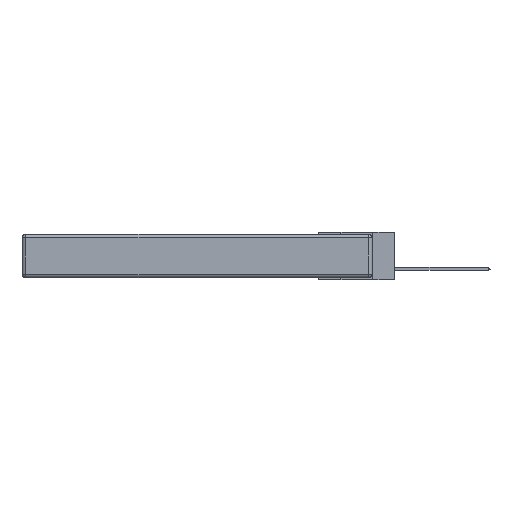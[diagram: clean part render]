
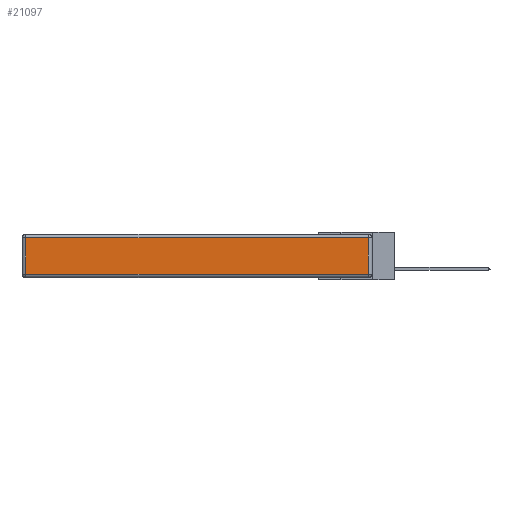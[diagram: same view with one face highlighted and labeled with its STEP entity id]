
A CAD part, left-side view. The second image highlights one B-rep face of the part: STEP entity #21097.
In plain terms, the highlighted planar face has unit normal (-1, 0, 0).
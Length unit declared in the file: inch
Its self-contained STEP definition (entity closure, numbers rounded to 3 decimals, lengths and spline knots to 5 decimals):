
#243 = EDGE_CURVE ( 'NONE', #16409, #22165, #5849, .T. ) ;
#747 = VERTEX_POINT ( 'NONE', #2492 ) ;
#1252 = AXIS2_PLACEMENT_3D ( 'NONE', #21568, #6762, #8653 ) ;
#2492 = CARTESIAN_POINT ( 'NONE',  ( 0., 0.03, -0.313 ) ) ;
#2910 = VECTOR ( 'NONE', #4854, 39.37008 ) ;
#4437 = CARTESIAN_POINT ( 'NONE',  ( 0., 0., -0.313 ) ) ;
#4854 = DIRECTION ( 'NONE',  ( 0., -1., 0. ) ) ;
#5485 = FACE_OUTER_BOUND ( 'NONE', #18201, .T. ) ;
#5849 = LINE ( 'NONE', #16202, #8765 ) ;
#6510 = CARTESIAN_POINT ( 'NONE',  ( 0., 2.75, -0.03 ) ) ;
#6762 = DIRECTION ( 'NONE',  ( -1., 0., 0. ) ) ;
#7307 = VECTOR ( 'NONE', #8206, 39.37008 ) ;
#8121 = ORIENTED_EDGE ( 'NONE', *, *, #243, .T. ) ;
#8206 = DIRECTION ( 'NONE',  ( 0., 0., 1. ) ) ;
#8380 = CARTESIAN_POINT ( 'NONE',  ( 0., 2.72, -0.313 ) ) ;
#8384 = EDGE_CURVE ( 'NONE', #22165, #747, #23804, .T. ) ;
#8400 = DIRECTION ( 'NONE',  ( 0., 1., 0. ) ) ;
#8653 = DIRECTION ( 'NONE',  ( 0., 0., 1. ) ) ;
#8765 = VECTOR ( 'NONE', #20094, 39.37008 ) ;
#10004 = EDGE_CURVE ( 'NONE', #747, #18647, #22603, .T. ) ;
#11236 = VECTOR ( 'NONE', #8400, 39.37008 ) ;
#13705 = CARTESIAN_POINT ( 'NONE',  ( 0., 0.03, -0.343 ) ) ;
#14139 = PLANE ( 'NONE',  #1252 ) ;
#15272 = ORIENTED_EDGE ( 'NONE', *, *, #8384, .T. ) ;
#16202 = CARTESIAN_POINT ( 'NONE',  ( 0., 2.72, -0.343 ) ) ;
#16280 = CARTESIAN_POINT ( 'NONE',  ( 0., 0.03, -0.03 ) ) ;
#16409 = VERTEX_POINT ( 'NONE', #20527 ) ;
#17378 = LINE ( 'NONE', #6510, #11236 ) ;
#17564 = EDGE_CURVE ( 'NONE', #18647, #16409, #17378, .T. ) ;
#17737 = ORIENTED_EDGE ( 'NONE', *, *, #17564, .T. ) ;
#18201 = EDGE_LOOP ( 'NONE', ( #15272, #19246, #17737, #8121 ) ) ;
#18647 = VERTEX_POINT ( 'NONE', #16280 ) ;
#19246 = ORIENTED_EDGE ( 'NONE', *, *, #10004, .T. ) ;
#20094 = DIRECTION ( 'NONE',  ( 0., 0., -1. ) ) ;
#20527 = CARTESIAN_POINT ( 'NONE',  ( 0., 2.72, -0.03 ) ) ;
#21097 = ADVANCED_FACE ( 'NONE', ( #5485 ), #14139, .T. ) ;
#21568 = CARTESIAN_POINT ( 'NONE',  ( 0., 0., -0.343 ) ) ;
#22165 = VERTEX_POINT ( 'NONE', #8380 ) ;
#22603 = LINE ( 'NONE', #13705, #7307 ) ;
#23804 = LINE ( 'NONE', #4437, #2910 ) ;
